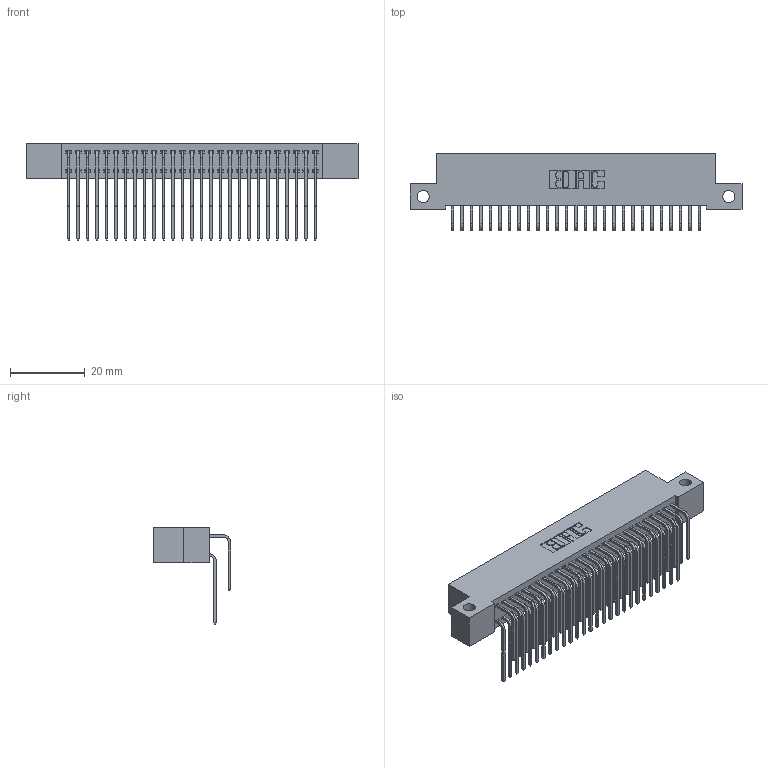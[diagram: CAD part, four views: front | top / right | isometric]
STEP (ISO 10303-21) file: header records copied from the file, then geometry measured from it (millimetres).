
FILE_DESCRIPTION (( 'STEP AP203' ), '1' );
FILE_NAME ('392-054-559-212.STEP', '2019-10-08T14:14:48', ( '' ), ( '' ), 'SwSTEP 2.0', 'SolidWorks 2016', '' );
FILE_SCHEMA (( 'CONFIG_CONTROL_DESIGN' ));
Length unit declared in the file: inch
Products named in the file (4): 342 Part_Side Mount; 345-292-001_558 559 Tail - 1; 345-292-001_559 Tail - 2; 392-054-559-212
Assembly tree (55 placements, depth 2):
  392-054-559-212
    342 Part_Side Mount
    345-292-001_558 559 Tail - 1  x27
    345-292-001_559 Tail - 2  x27
Bounding box: 88.9 x 20.64 x 25.78 mm (x, y, z)
Volume: 8154.2 mm3; surface area: 14152.8 mm2
Topology: 55 solids, 55 shells, 3026 faces, 8993 edges, 5922 vertices
Faces by surface type: plane 2118, cylinder 908
Entity records: 20965 total; most frequent: CARTESIAN_POINT 3541, ORIENTED_EDGE 3426, DIRECTION 3033, EDGE_CURVE 1713, VECTOR 1545, LINE 1545, VERTEX_POINT 1138, AXIS2_PLACEMENT_3D 744
